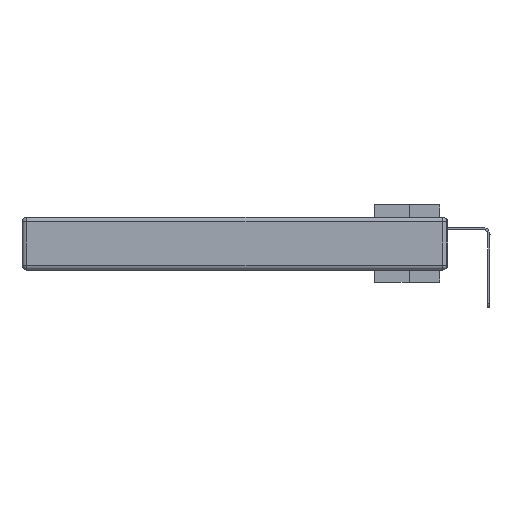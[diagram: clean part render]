
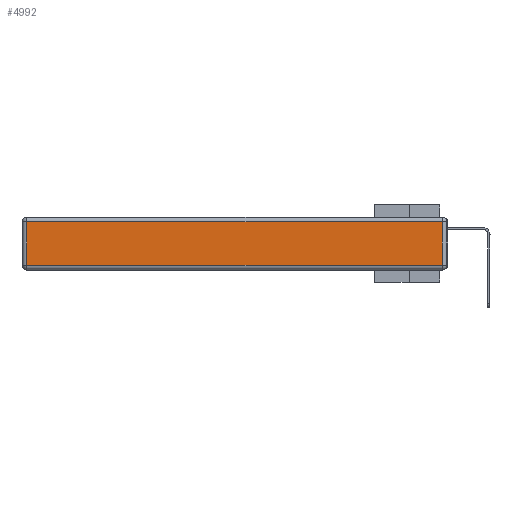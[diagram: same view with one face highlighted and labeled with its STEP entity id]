
A CAD part, left-side view. The second image highlights one B-rep face of the part: STEP entity #4992.
In plain terms, the highlighted planar face has unit normal (-1, 0, 0).
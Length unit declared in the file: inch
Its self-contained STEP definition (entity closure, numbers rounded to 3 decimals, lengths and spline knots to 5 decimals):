
#934 = VERTEX_POINT ( 'NONE', #23084 ) ;
#1611 = ORIENTED_EDGE ( 'NONE', *, *, #10987, .T. ) ;
#2535 = DIRECTION ( 'NONE',  ( -1., 0., 0. ) ) ;
#3257 = ORIENTED_EDGE ( 'NONE', *, *, #7023, .T. ) ;
#4267 = EDGE_CURVE ( 'NONE', #5106, #934, #33373, .T. ) ;
#4636 = VECTOR ( 'NONE', #17849, 39.37008 ) ;
#4809 = FACE_OUTER_BOUND ( 'NONE', #22994, .T. ) ;
#4969 = CARTESIAN_POINT ( 'NONE',  ( 0., 2.72, -0.343 ) ) ;
#4992 = ADVANCED_FACE ( 'NONE', ( #4809 ), #18241, .T. ) ;
#5106 = VERTEX_POINT ( 'NONE', #10369 ) ;
#6892 = LINE ( 'NONE', #14213, #14180 ) ;
#7023 = EDGE_CURVE ( 'NONE', #22473, #16217, #16846, .T. ) ;
#7745 = CARTESIAN_POINT ( 'NONE',  ( 0., 2.72, -0.313 ) ) ;
#8109 = DIRECTION ( 'NONE',  ( 0., 0., 1. ) ) ;
#8509 = ORIENTED_EDGE ( 'NONE', *, *, #12159, .T. ) ;
#10369 = CARTESIAN_POINT ( 'NONE',  ( 0., 0.03, -0.313 ) ) ;
#10536 = VECTOR ( 'NONE', #20004, 39.37008 ) ;
#10987 = EDGE_CURVE ( 'NONE', #934, #22473, #6892, .T. ) ;
#11709 = DIRECTION ( 'NONE',  ( 0., 1., 0. ) ) ;
#12159 = EDGE_CURVE ( 'NONE', #16217, #5106, #32481, .T. ) ;
#14180 = VECTOR ( 'NONE', #11709, 39.37008 ) ;
#14213 = CARTESIAN_POINT ( 'NONE',  ( 0., 2.75, -0.03 ) ) ;
#14937 = VECTOR ( 'NONE', #21930, 39.37008 ) ;
#16217 = VERTEX_POINT ( 'NONE', #7745 ) ;
#16674 = CARTESIAN_POINT ( 'NONE',  ( 0., 0., -0.313 ) ) ;
#16846 = LINE ( 'NONE', #4969, #4636 ) ;
#17849 = DIRECTION ( 'NONE',  ( 0., 0., -1. ) ) ;
#18241 = PLANE ( 'NONE',  #26401 ) ;
#18490 = ORIENTED_EDGE ( 'NONE', *, *, #4267, .T. ) ;
#20004 = DIRECTION ( 'NONE',  ( 0., 0., 1. ) ) ;
#21930 = DIRECTION ( 'NONE',  ( 0., -1., 0. ) ) ;
#22473 = VERTEX_POINT ( 'NONE', #31019 ) ;
#22994 = EDGE_LOOP ( 'NONE', ( #8509, #18490, #1611, #3257 ) ) ;
#23084 = CARTESIAN_POINT ( 'NONE',  ( 0., 0.03, -0.03 ) ) ;
#25461 = CARTESIAN_POINT ( 'NONE',  ( 0., 0.03, -0.343 ) ) ;
#26401 = AXIS2_PLACEMENT_3D ( 'NONE', #28706, #2535, #8109 ) ;
#28706 = CARTESIAN_POINT ( 'NONE',  ( 0., 0., -0.343 ) ) ;
#31019 = CARTESIAN_POINT ( 'NONE',  ( 0., 2.72, -0.03 ) ) ;
#32481 = LINE ( 'NONE', #16674, #14937 ) ;
#33373 = LINE ( 'NONE', #25461, #10536 ) ;
